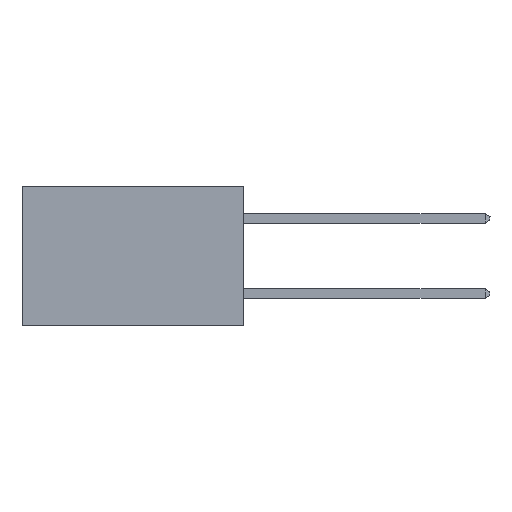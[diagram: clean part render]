
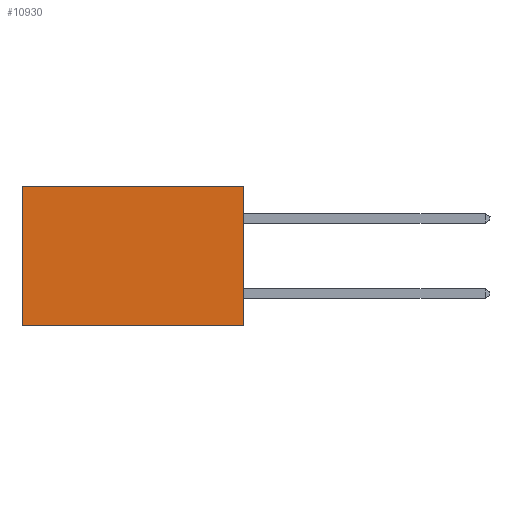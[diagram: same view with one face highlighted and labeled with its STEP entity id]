
A CAD part, left-side view. The second image highlights one B-rep face of the part: STEP entity #10930.
In plain terms, the highlighted planar face has unit normal (-1, 0, 0).
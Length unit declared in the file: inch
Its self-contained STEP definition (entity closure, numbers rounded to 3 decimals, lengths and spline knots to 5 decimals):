
#254 = EDGE_CURVE ( 'NONE', #14006, #7387, #1473, .T. ) ;
#334 = DIRECTION ( 'NONE',  ( 0., 0., -1. ) ) ;
#515 = CARTESIAN_POINT ( 'NONE',  ( 0.277, 0.59, -0.37 ) ) ;
#547 = LINE ( 'NONE', #16029, #7081 ) ;
#963 = VERTEX_POINT ( 'NONE', #2959 ) ;
#1448 = EDGE_LOOP ( 'NONE', ( #10542, #11255, #11590, #11636 ) ) ;
#1473 = LINE ( 'NONE', #1633, #7973 ) ;
#1549 = AXIS2_PLACEMENT_3D ( 'NONE', #11300, #3789, #12553 ) ;
#1633 = CARTESIAN_POINT ( 'NONE',  ( 0.277, 0., 0. ) ) ;
#2703 = EDGE_CURVE ( 'NONE', #14006, #963, #2808, .T. ) ;
#2808 = LINE ( 'NONE', #5226, #15826 ) ;
#2959 = CARTESIAN_POINT ( 'NONE',  ( 0.277, 0., -0.37 ) ) ;
#2998 = DIRECTION ( 'NONE',  ( 0., 0., -1. ) ) ;
#3575 = VERTEX_POINT ( 'NONE', #13225 ) ;
#3789 = DIRECTION ( 'NONE',  ( 1., 0., 0. ) ) ;
#5226 = CARTESIAN_POINT ( 'NONE',  ( 0.277, 0., -0.37 ) ) ;
#6191 = FACE_OUTER_BOUND ( 'NONE', #1448, .T. ) ;
#6952 = VECTOR ( 'NONE', #334, 39.37008 ) ;
#7081 = VECTOR ( 'NONE', #7394, 39.37008 ) ;
#7387 = VERTEX_POINT ( 'NONE', #13671 ) ;
#7394 = DIRECTION ( 'NONE',  ( 0., 1., 0. ) ) ;
#7743 = EDGE_CURVE ( 'NONE', #7387, #3575, #10612, .T. ) ;
#7973 = VECTOR ( 'NONE', #15254, 39.37008 ) ;
#10542 = ORIENTED_EDGE ( 'NONE', *, *, #7743, .T. ) ;
#10612 = LINE ( 'NONE', #515, #6952 ) ;
#10930 = ADVANCED_FACE ( 'NONE', ( #6191 ), #13766, .F. ) ;
#11255 = ORIENTED_EDGE ( 'NONE', *, *, #14675, .F. ) ;
#11300 = CARTESIAN_POINT ( 'NONE',  ( 0.277, 0., -0.37 ) ) ;
#11590 = ORIENTED_EDGE ( 'NONE', *, *, #2703, .F. ) ;
#11636 = ORIENTED_EDGE ( 'NONE', *, *, #254, .T. ) ;
#12553 = DIRECTION ( 'NONE',  ( 0., 0., -1. ) ) ;
#13225 = CARTESIAN_POINT ( 'NONE',  ( 0.277, 0.59, -0.37 ) ) ;
#13671 = CARTESIAN_POINT ( 'NONE',  ( 0.277, 0.59, 0. ) ) ;
#13766 = PLANE ( 'NONE',  #1549 ) ;
#14006 = VERTEX_POINT ( 'NONE', #14695 ) ;
#14675 = EDGE_CURVE ( 'NONE', #963, #3575, #547, .T. ) ;
#14695 = CARTESIAN_POINT ( 'NONE',  ( 0.277, 0., 0. ) ) ;
#15254 = DIRECTION ( 'NONE',  ( 0., 1., 0. ) ) ;
#15826 = VECTOR ( 'NONE', #2998, 39.37008 ) ;
#16029 = CARTESIAN_POINT ( 'NONE',  ( 0.277, 0., -0.37 ) ) ;
